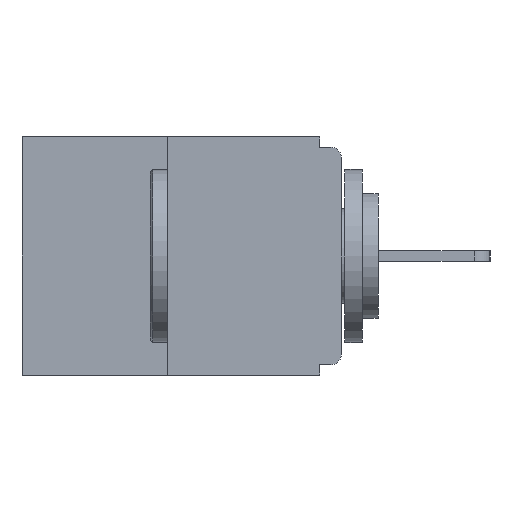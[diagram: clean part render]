
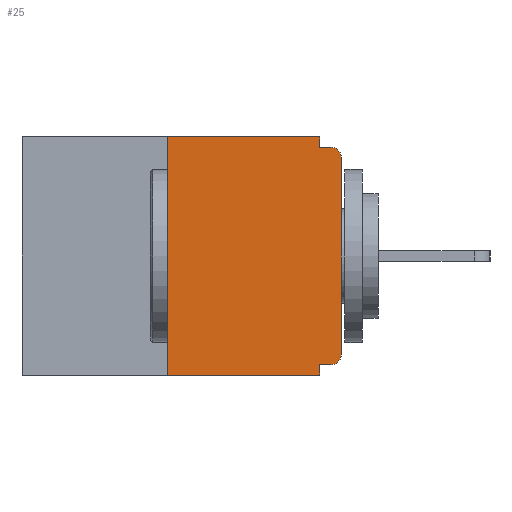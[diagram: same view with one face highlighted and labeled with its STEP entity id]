
A CAD part, left-side view. The second image highlights one B-rep face of the part: STEP entity #25.
In plain terms, the highlighted planar face has unit normal (-1, 0, 0).
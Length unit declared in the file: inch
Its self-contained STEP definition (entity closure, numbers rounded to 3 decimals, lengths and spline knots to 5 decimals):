
#25 = ADVANCED_FACE ( 'NONE', ( #18597 ), #10786, .F. ) ;
#826 = DIRECTION ( 'NONE',  ( -1., 0., 0. ) ) ;
#924 = DIRECTION ( 'NONE',  ( 0., -1., 0. ) ) ;
#989 = VERTEX_POINT ( 'NONE', #19283 ) ;
#1012 = CARTESIAN_POINT ( 'NONE',  ( 0., 0.46, -0.343 ) ) ;
#1248 = VERTEX_POINT ( 'NONE', #18490 ) ;
#1275 = AXIS2_PLACEMENT_3D ( 'NONE', #20726, #10205, #25553 ) ;
#1686 = DIRECTION ( 'NONE',  ( 0., 0., -1. ) ) ;
#1779 = EDGE_CURVE ( 'NONE', #5567, #989, #4462, .T. ) ;
#2142 = EDGE_CURVE ( 'NONE', #1248, #21189, #11632, .T. ) ;
#2424 = VECTOR ( 'NONE', #16855, 39.37008 ) ;
#2715 = LINE ( 'NONE', #22370, #13390 ) ;
#3059 = VERTEX_POINT ( 'NONE', #13805 ) ;
#3190 = EDGE_CURVE ( 'NONE', #5567, #17728, #13120, .T. ) ;
#3773 = CARTESIAN_POINT ( 'NONE',  ( 0., 0., -0.313 ) ) ;
#3887 = CARTESIAN_POINT ( 'NONE',  ( 0., 0.031, -0.015 ) ) ;
#3895 = EDGE_CURVE ( 'NONE', #17728, #3059, #2715, .T. ) ;
#4185 = VERTEX_POINT ( 'NONE', #14725 ) ;
#4462 = LINE ( 'NONE', #1012, #14461 ) ;
#4965 = CARTESIAN_POINT ( 'NONE',  ( 0., 0., -0.328 ) ) ;
#5364 = CARTESIAN_POINT ( 'NONE',  ( 0., 0.031, 0. ) ) ;
#5567 = VERTEX_POINT ( 'NONE', #20382 ) ;
#5694 = ORIENTED_EDGE ( 'NONE', *, *, #3895, .F. ) ;
#5747 = ORIENTED_EDGE ( 'NONE', *, *, #3190, .F. ) ;
#5897 = ORIENTED_EDGE ( 'NONE', *, *, #1779, .T. ) ;
#6047 = CARTESIAN_POINT ( 'NONE',  ( 0., 0.031, -0.343 ) ) ;
#6133 = ORIENTED_EDGE ( 'NONE', *, *, #24842, .F. ) ;
#6278 = LINE ( 'NONE', #5364, #21422 ) ;
#6417 = ORIENTED_EDGE ( 'NONE', *, *, #2142, .F. ) ;
#6705 = ORIENTED_EDGE ( 'NONE', *, *, #18781, .T. ) ;
#6835 = ORIENTED_EDGE ( 'NONE', *, *, #8984, .T. ) ;
#6911 = ORIENTED_EDGE ( 'NONE', *, *, #16195, .T. ) ;
#7007 = ORIENTED_EDGE ( 'NONE', *, *, #22626, .F. ) ;
#7113 = ORIENTED_EDGE ( 'NONE', *, *, #22310, .F. ) ;
#7436 = DIRECTION ( 'NONE',  ( 0., 0., -1. ) ) ;
#8144 = LINE ( 'NONE', #22522, #18087 ) ;
#8491 = DIRECTION ( 'NONE',  ( 0., 0., 1. ) ) ;
#8968 = CIRCLE ( 'NONE', #11434, 0.015 ) ;
#8984 = EDGE_CURVE ( 'NONE', #15830, #19594, #24569, .T. ) ;
#9856 = CARTESIAN_POINT ( 'NONE',  ( 0., 0.25, 0. ) ) ;
#10205 = DIRECTION ( 'NONE',  ( 1., 0., 0. ) ) ;
#10721 = CIRCLE ( 'NONE', #24147, 0.015 ) ;
#10786 = PLANE ( 'NONE',  #1275 ) ;
#11433 = VECTOR ( 'NONE', #11941, 39.37008 ) ;
#11434 = AXIS2_PLACEMENT_3D ( 'NONE', #25384, #13755, #1686 ) ;
#11632 = LINE ( 'NONE', #4965, #22095 ) ;
#11941 = DIRECTION ( 'NONE',  ( 0., 0., -1. ) ) ;
#12448 = CARTESIAN_POINT ( 'NONE',  ( 0., 0., 0. ) ) ;
#12748 = DIRECTION ( 'NONE',  ( 0., -1., 0. ) ) ;
#12944 = CARTESIAN_POINT ( 'NONE',  ( 0., 0.015, -0.03 ) ) ;
#13120 = LINE ( 'NONE', #16936, #2424 ) ;
#13390 = VECTOR ( 'NONE', #24083, 39.37008 ) ;
#13755 = DIRECTION ( 'NONE',  ( -1., 0., 0. ) ) ;
#13805 = CARTESIAN_POINT ( 'NONE',  ( 0., 0.031, 0. ) ) ;
#14341 = CARTESIAN_POINT ( 'NONE',  ( 0., 0., -0.03 ) ) ;
#14348 = EDGE_LOOP ( 'NONE', ( #5694, #5747, #5897, #6133, #6417, #6705, #6835, #6911, #7007, #7113 ) ) ;
#14461 = VECTOR ( 'NONE', #924, 39.37008 ) ;
#14725 = CARTESIAN_POINT ( 'NONE',  ( 0., 0.015, -0.015 ) ) ;
#14982 = DIRECTION ( 'NONE',  ( 0., 0., -1. ) ) ;
#15830 = VERTEX_POINT ( 'NONE', #3773 ) ;
#16195 = EDGE_CURVE ( 'NONE', #19594, #4185, #10721, .T. ) ;
#16855 = DIRECTION ( 'NONE',  ( 0., 0., 1. ) ) ;
#16936 = CARTESIAN_POINT ( 'NONE',  ( 0., 0.25, 0. ) ) ;
#17400 = LINE ( 'NONE', #6047, #11433 ) ;
#17728 = VERTEX_POINT ( 'NONE', #9856 ) ;
#18087 = VECTOR ( 'NONE', #12748, 39.37008 ) ;
#18490 = CARTESIAN_POINT ( 'NONE',  ( 0., 0.015, -0.328 ) ) ;
#18597 = FACE_OUTER_BOUND ( 'NONE', #14348, .T. ) ;
#18781 = EDGE_CURVE ( 'NONE', #1248, #15830, #8968, .T. ) ;
#19283 = CARTESIAN_POINT ( 'NONE',  ( 0., 0.031, -0.343 ) ) ;
#19594 = VERTEX_POINT ( 'NONE', #14341 ) ;
#20382 = CARTESIAN_POINT ( 'NONE',  ( 0., 0.25, -0.343 ) ) ;
#20726 = CARTESIAN_POINT ( 'NONE',  ( 0., 0.46, 0. ) ) ;
#21189 = VERTEX_POINT ( 'NONE', #23290 ) ;
#21422 = VECTOR ( 'NONE', #7436, 39.37008 ) ;
#22095 = VECTOR ( 'NONE', #22992, 39.37008 ) ;
#22310 = EDGE_CURVE ( 'NONE', #3059, #22937, #6278, .T. ) ;
#22370 = CARTESIAN_POINT ( 'NONE',  ( 0., 0.46, 0. ) ) ;
#22522 = CARTESIAN_POINT ( 'NONE',  ( 0., 0., -0.015 ) ) ;
#22626 = EDGE_CURVE ( 'NONE', #22937, #4185, #8144, .T. ) ;
#22937 = VERTEX_POINT ( 'NONE', #3887 ) ;
#22992 = DIRECTION ( 'NONE',  ( 0., 1., 0. ) ) ;
#23290 = CARTESIAN_POINT ( 'NONE',  ( 0., 0.031, -0.328 ) ) ;
#24083 = DIRECTION ( 'NONE',  ( 0., -1., 0. ) ) ;
#24147 = AXIS2_PLACEMENT_3D ( 'NONE', #12944, #826, #14982 ) ;
#24569 = LINE ( 'NONE', #12448, #25176 ) ;
#24842 = EDGE_CURVE ( 'NONE', #21189, #989, #17400, .T. ) ;
#25176 = VECTOR ( 'NONE', #8491, 39.37008 ) ;
#25384 = CARTESIAN_POINT ( 'NONE',  ( 0., 0.015, -0.313 ) ) ;
#25553 = DIRECTION ( 'NONE',  ( 0., 0., -1. ) ) ;
